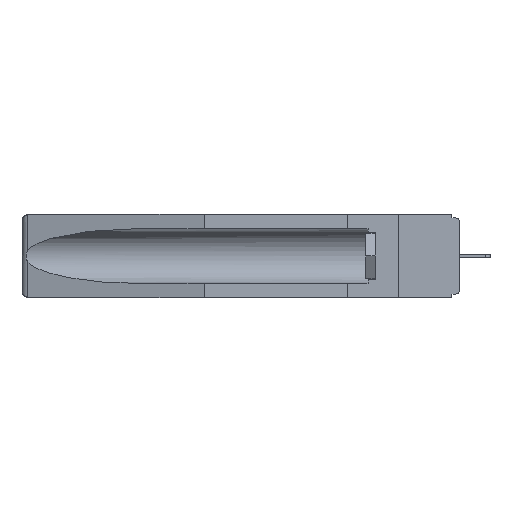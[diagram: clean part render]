
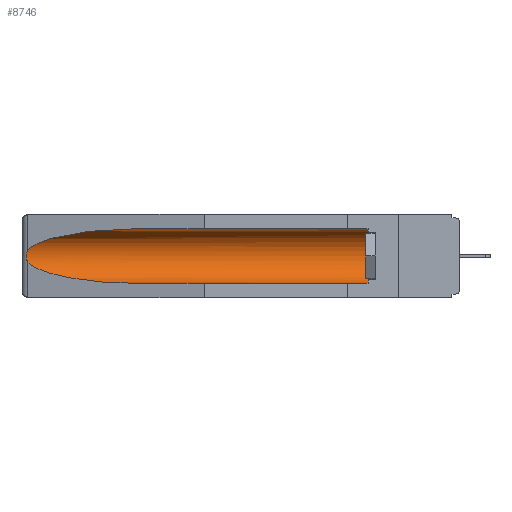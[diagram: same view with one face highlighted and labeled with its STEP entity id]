
A CAD part, left-side view. The second image highlights one B-rep face of the part: STEP entity #8746.
In plain terms, the highlighted cylindrical face has radius 2.857 mm (diameter 5.715 mm), a partial arc.
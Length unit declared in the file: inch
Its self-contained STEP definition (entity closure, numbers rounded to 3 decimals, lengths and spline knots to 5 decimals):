
#54 = EDGE_CURVE ( 'NONE', #6709, #15317, #11650, .T. ) ;
#69 = CARTESIAN_POINT ( 'NONE',  ( 0.155, 1.07973, -0.284 ) ) ;
#248 = CARTESIAN_POINT ( 'NONE',  ( 0.155, -0.30754, -0.059 ) ) ;
#416 = CARTESIAN_POINT ( 'NONE',  ( 0.26537, 1.52718, -0.19328 ) ) ;
#520 = CARTESIAN_POINT ( 'NONE',  ( 0.155, 0.126, -0.284 ) ) ;
#600 = CARTESIAN_POINT ( 'NONE',  ( 0.2675, 1.53308, -0.17534 ) ) ;
#869 = LINE ( 'NONE', #248, #15099 ) ;
#1003 = ORIENTED_EDGE ( 'NONE', *, *, #9917, .T. ) ;
#2349 = ORIENTED_EDGE ( 'NONE', *, *, #5378, .T. ) ;
#2848 = B_SPLINE_CURVE_WITH_KNOTS ( 'NONE', 3,
 ( #2903, #7554, #15968, #16340, #7639, #600, #16066, #3277, #10701, #416 ),
 .UNSPECIFIED., .F., .F.,
 ( 4, 2, 2, 2, 4 ),
 ( 0., 0.00029, 0.00058, 0.00087, 0.00117 ),
 .UNSPECIFIED. ) ;
#2903 = CARTESIAN_POINT ( 'NONE',  ( 0.26537, 1.52718, -0.14972 ) ) ;
#2983 = ORIENTED_EDGE ( 'NONE', *, *, #6954, .T. ) ;
#3277 = CARTESIAN_POINT ( 'NONE',  ( 0.26655, 1.53094, -0.18657 ) ) ;
#5212 = VERTEX_POINT ( 'NONE', #8224 ) ;
#5378 = EDGE_CURVE ( 'NONE', #15317, #12805, #869, .T. ) ;
#5627 = CARTESIAN_POINT ( 'NONE',  ( 0.155, 1.07973, -0.059 ) ) ;
#6199 = CARTESIAN_POINT ( 'NONE',  ( 0.21114, 1.30732, -0.284 ) ) ;
#6457 = LINE ( 'NONE', #15209, #11129 ) ;
#6709 = VERTEX_POINT ( 'NONE', #520 ) ;
#6954 = EDGE_CURVE ( 'NONE', #12805, #18036, #18192, .T. ) ;
#7016 = VERTEX_POINT ( 'NONE', #69 ) ;
#7113 = CARTESIAN_POINT ( 'NONE',  ( 0.25451, 1.48313, -0.09465 ) ) ;
#7122 = CARTESIAN_POINT ( 'NONE',  ( 0.155, 1.07973, -0.059 ) ) ;
#7386 = CARTESIAN_POINT ( 'NONE',  ( 0.26537, 1.52718, -0.14972 ) ) ;
#7554 = CARTESIAN_POINT ( 'NONE',  ( 0.26597, 1.52961, -0.15275 ) ) ;
#7639 = CARTESIAN_POINT ( 'NONE',  ( 0.2675, 1.53308, -0.16763 ) ) ;
#8224 = CARTESIAN_POINT ( 'NONE',  ( 0.26537, 1.52718, -0.19328 ) ) ;
#8521 = EDGE_LOOP ( 'NONE', ( #2983, #1003, #16956, #9727, #11005, #2349 ) ) ;
#8746 = ADVANCED_FACE ( 'NONE', ( #8953 ), #14747, .F. ) ;
#8806 = CARTESIAN_POINT ( 'NONE',  ( 0.155, 1.07973, -0.284 ) ) ;
#8953 = FACE_OUTER_BOUND ( 'NONE', #8521, .T. ) ;
#9572 =( BOUNDED_CURVE ( )  B_SPLINE_CURVE ( 3, ( #15834, #13139, #6199, #8806 ),
 .UNSPECIFIED., .F., .F. ) 
 B_SPLINE_CURVE_WITH_KNOTS ( ( 4, 4 ),
 ( 0.1948, 1.5708 ),
 .UNSPECIFIED. ) 
 CURVE ( )  GEOMETRIC_REPRESENTATION_ITEM ( )  RATIONAL_B_SPLINE_CURVE ( ( 1., 0.848, 0.848, 1. ) ) 
 REPRESENTATION_ITEM ( '' )  );
#9727 = ORIENTED_EDGE ( 'NONE', *, *, #11805, .F. ) ;
#9879 = AXIS2_PLACEMENT_3D ( 'NONE', #11436, #17058, #10040 ) ;
#9917 = EDGE_CURVE ( 'NONE', #18036, #5212, #2848, .T. ) ;
#10040 = DIRECTION ( 'NONE',  ( 0., 0., 1. ) ) ;
#10331 = CARTESIAN_POINT ( 'NONE',  ( 0.155, -0.30754, -0.1715 ) ) ;
#10701 = CARTESIAN_POINT ( 'NONE',  ( 0.26597, 1.5296, -0.19026 ) ) ;
#10785 = DIRECTION ( 'NONE',  ( 0., 1., 0. ) ) ;
#11005 = ORIENTED_EDGE ( 'NONE', *, *, #54, .T. ) ;
#11129 = VECTOR ( 'NONE', #13819, 39.37008 ) ;
#11390 = CARTESIAN_POINT ( 'NONE',  ( 0.155, 0.126, -0.059 ) ) ;
#11436 = CARTESIAN_POINT ( 'NONE',  ( 0.155, 0.126, -0.1715 ) ) ;
#11650 = CIRCLE ( 'NONE', #9879, 0.1125 ) ;
#11654 = CARTESIAN_POINT ( 'NONE',  ( 0.21114, 1.30732, -0.059 ) ) ;
#11805 = EDGE_CURVE ( 'NONE', #6709, #7016, #6457, .T. ) ;
#12805 = VERTEX_POINT ( 'NONE', #7122 ) ;
#13139 = CARTESIAN_POINT ( 'NONE',  ( 0.25451, 1.48313, -0.24835 ) ) ;
#13819 = DIRECTION ( 'NONE',  ( 0., 1., 0. ) ) ;
#14747 = CYLINDRICAL_SURFACE ( 'NONE', #16973, 0.1125 ) ;
#14775 = CARTESIAN_POINT ( 'NONE',  ( 0.26537, 1.52718, -0.14972 ) ) ;
#14946 = EDGE_CURVE ( 'NONE', #5212, #7016, #9572, .T. ) ;
#15099 = VECTOR ( 'NONE', #10785, 39.37008 ) ;
#15209 = CARTESIAN_POINT ( 'NONE',  ( 0.155, -0.30754, -0.284 ) ) ;
#15317 = VERTEX_POINT ( 'NONE', #11390 ) ;
#15834 = CARTESIAN_POINT ( 'NONE',  ( 0.26537, 1.52718, -0.19328 ) ) ;
#15964 = DIRECTION ( 'NONE',  ( 0., 0., 1. ) ) ;
#15968 = CARTESIAN_POINT ( 'NONE',  ( 0.26654, 1.53092, -0.15636 ) ) ;
#16066 = CARTESIAN_POINT ( 'NONE',  ( 0.2673, 1.53269, -0.17917 ) ) ;
#16340 = CARTESIAN_POINT ( 'NONE',  ( 0.2673, 1.5327, -0.16383 ) ) ;
#16956 = ORIENTED_EDGE ( 'NONE', *, *, #14946, .T. ) ;
#16973 = AXIS2_PLACEMENT_3D ( 'NONE', #10331, #17715, #15964 ) ;
#17058 = DIRECTION ( 'NONE',  ( 0., -1., 0. ) ) ;
#17715 = DIRECTION ( 'NONE',  ( 0., 1., 0. ) ) ;
#18036 = VERTEX_POINT ( 'NONE', #14775 ) ;
#18192 =( BOUNDED_CURVE ( )  B_SPLINE_CURVE ( 3, ( #5627, #11654, #7113, #7386 ),
 .UNSPECIFIED., .F., .F. ) 
 B_SPLINE_CURVE_WITH_KNOTS ( ( 4, 4 ),
 ( 4.71239, 6.08839 ),
 .UNSPECIFIED. ) 
 CURVE ( )  GEOMETRIC_REPRESENTATION_ITEM ( )  RATIONAL_B_SPLINE_CURVE ( ( 1., 0.848, 0.848, 1. ) ) 
 REPRESENTATION_ITEM ( '' )  );
